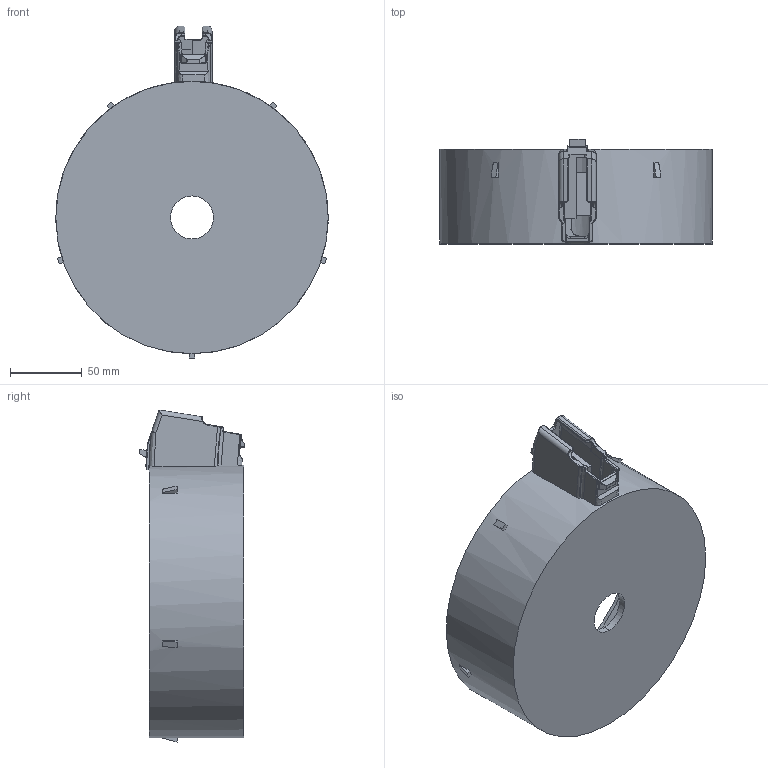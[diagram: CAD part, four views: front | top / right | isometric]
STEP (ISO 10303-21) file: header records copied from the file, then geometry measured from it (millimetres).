
FILE_DESCRIPTION (( 'STEP AP203' ), '1' );
FILE_NAME ('front.STEP', '2013-09-09T02:38:38', ( '' ), ( '' ), 'SwSTEP 2.0', 'SolidWorks 2013', '' );
FILE_SCHEMA (( 'CONFIG_CONTROL_DESIGN' ));
Length unit declared in the file: millimetre
Products named in the file (1): front
Bounding box: 190 x 73.71 x 231.56 mm (x, y, z)
Volume: 391341.7 mm3; surface area: 169564.3 mm2
Topology: 1 solids, 1 shells, 334 faces, 857 edges, 517 vertices
Faces by surface type: cylinder 115, bspline 106, plane 92, torus 17, cone 4
Entity records: 15642 total; most frequent: CARTESIAN_POINT 8470, ORIENTED_EDGE 1688, DIRECTION 1236, EDGE_CURVE 844, VERTEX_POINT 517, AXIS2_PLACEMENT_3D 469, EDGE_LOOP 343, FACE_OUTER_BOUND 334
